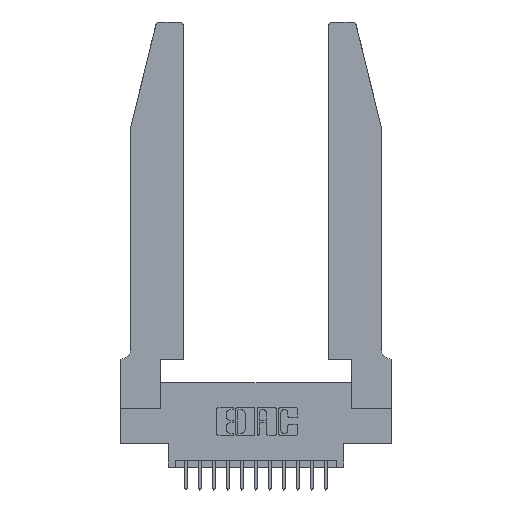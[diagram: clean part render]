
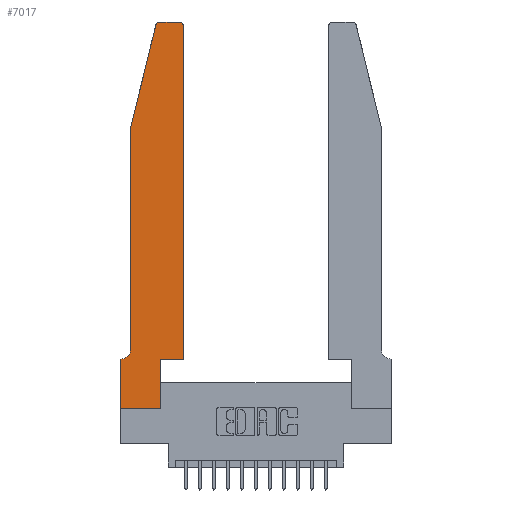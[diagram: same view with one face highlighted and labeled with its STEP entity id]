
A CAD part, top view. The second image highlights one B-rep face of the part: STEP entity #7017.
In plain terms, the highlighted planar face has unit normal (0, 0, 1).
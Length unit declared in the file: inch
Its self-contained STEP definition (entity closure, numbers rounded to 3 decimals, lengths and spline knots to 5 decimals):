
#17 = EDGE_CURVE ( 'NONE', #16693, #17585, #17739, .T. ) ;
#855 = CARTESIAN_POINT ( 'NONE',  ( 0.4505, 2.72, 0.37 ) ) ;
#924 = CARTESIAN_POINT ( 'NONE',  ( 0., 0., 0.37 ) ) ;
#1266 = CARTESIAN_POINT ( 'NONE',  ( 0.0755, 2., 0.37 ) ) ;
#1365 = CARTESIAN_POINT ( 'NONE',  ( 0.284, 2.75, 0.37 ) ) ;
#1381 = CARTESIAN_POINT ( 'NONE',  ( 0.4505, 0.35, 0.37 ) ) ;
#1466 = EDGE_CURVE ( 'NONE', #13858, #3915, #9994, .T. ) ;
#1896 = DIRECTION ( 'NONE',  ( 1., 0., 0. ) ) ;
#2001 = CARTESIAN_POINT ( 'NONE',  ( 0., 0., 0.37 ) ) ;
#2240 = DIRECTION ( 'NONE',  ( 0., 0., 1. ) ) ;
#2262 = DIRECTION ( 'NONE',  ( 0., 1., 0. ) ) ;
#3110 = CARTESIAN_POINT ( 'NONE',  ( 0.0755, 2., 0.37 ) ) ;
#3193 = ORIENTED_EDGE ( 'NONE', *, *, #17, .T. ) ;
#3297 = PLANE ( 'NONE',  #13897 ) ;
#3320 = DIRECTION ( 'NONE',  ( 1., 0., 0. ) ) ;
#3636 = ORIENTED_EDGE ( 'NONE', *, *, #8196, .T. ) ;
#3915 = VERTEX_POINT ( 'NONE', #15317 ) ;
#4298 = VERTEX_POINT ( 'NONE', #10493 ) ;
#4442 = CARTESIAN_POINT ( 'NONE',  ( 0.2865, 0., 0.37 ) ) ;
#4523 = CIRCLE ( 'NONE', #15562, 0.03 ) ;
#4702 = DIRECTION ( 'NONE',  ( 0., 0., 1. ) ) ;
#4775 = CARTESIAN_POINT ( 'NONE',  ( 0., 0.35, 0.37 ) ) ;
#5128 = LINE ( 'NONE', #2001, #5768 ) ;
#5158 = DIRECTION ( 'NONE',  ( -1., 0., 0. ) ) ;
#5293 = ORIENTED_EDGE ( 'NONE', *, *, #9450, .T. ) ;
#5401 = CARTESIAN_POINT ( 'NONE',  ( 0.2605, 2.75, 0.37 ) ) ;
#5768 = VECTOR ( 'NONE', #17195, 39.37008 ) ;
#6060 = LINE ( 'NONE', #14858, #16140 ) ;
#6226 = ORIENTED_EDGE ( 'NONE', *, *, #16073, .T. ) ;
#6567 = DIRECTION ( 'NONE',  ( 1., 0., 0. ) ) ;
#6626 = ORIENTED_EDGE ( 'NONE', *, *, #1466, .T. ) ;
#6933 = CARTESIAN_POINT ( 'NONE',  ( 0.4505, 0.35, 0.37 ) ) ;
#7017 = ADVANCED_FACE ( 'NONE', ( #11377 ), #3297, .T. ) ;
#7456 = DIRECTION ( 'NONE',  ( -1., 0., 0. ) ) ;
#7476 = EDGE_CURVE ( 'NONE', #12177, #15743, #13781, .T. ) ;
#7520 = DIRECTION ( 'NONE',  ( 1., 0., 0. ) ) ;
#7745 = VECTOR ( 'NONE', #3320, 39.37008 ) ;
#8021 = VECTOR ( 'NONE', #5158, 39.37008 ) ;
#8196 = EDGE_CURVE ( 'NONE', #17066, #16293, #16117, .T. ) ;
#8340 = ORIENTED_EDGE ( 'NONE', *, *, #13530, .T. ) ;
#8384 = LINE ( 'NONE', #16375, #7745 ) ;
#8445 = VERTEX_POINT ( 'NONE', #11913 ) ;
#8677 = DIRECTION ( 'NONE',  ( 0., 0., 1. ) ) ;
#8861 = EDGE_CURVE ( 'NONE', #15046, #17066, #13732, .T. ) ;
#8877 = DIRECTION ( 'NONE',  ( 0., 0., -1. ) ) ;
#8981 = ORIENTED_EDGE ( 'NONE', *, *, #7476, .T. ) ;
#9098 = CARTESIAN_POINT ( 'NONE',  ( 0.4205, 2.72, 0.37 ) ) ;
#9450 = EDGE_CURVE ( 'NONE', #15743, #16693, #5128, .T. ) ;
#9690 = CARTESIAN_POINT ( 'NONE',  ( 0., 0., 0.37 ) ) ;
#9819 = ORIENTED_EDGE ( 'NONE', *, *, #16255, .T. ) ;
#9908 = DIRECTION ( 'NONE',  ( 0., -1., 0. ) ) ;
#9994 = LINE ( 'NONE', #1266, #16200 ) ;
#10040 = CARTESIAN_POINT ( 'NONE',  ( 0.0055, 0.42, 0.37 ) ) ;
#10327 = DIRECTION ( 'NONE',  ( -1., 0., 0. ) ) ;
#10446 = AXIS2_PLACEMENT_3D ( 'NONE', #9098, #2240, #17386 ) ;
#10493 = CARTESIAN_POINT ( 'NONE',  ( 0.2865, 0.35, 0.37 ) ) ;
#10815 = DIRECTION ( 'NONE',  ( 0., 1., 0. ) ) ;
#11259 = AXIS2_PLACEMENT_3D ( 'NONE', #10040, #8877, #7456 ) ;
#11377 = FACE_OUTER_BOUND ( 'NONE', #15576, .T. ) ;
#11834 = VECTOR ( 'NONE', #10327, 39.37008 ) ;
#11913 = CARTESIAN_POINT ( 'NONE',  ( 0.25487, 2.72718, 0.37 ) ) ;
#11990 = ORIENTED_EDGE ( 'NONE', *, *, #8861, .T. ) ;
#12085 = ORIENTED_EDGE ( 'NONE', *, *, #14367, .T. ) ;
#12177 = VERTEX_POINT ( 'NONE', #16287 ) ;
#12669 = CARTESIAN_POINT ( 'NONE',  ( 0.0755, 0.35, 0.37 ) ) ;
#12782 = CARTESIAN_POINT ( 'NONE',  ( 0.284, 2.72, 0.37 ) ) ;
#12900 = CARTESIAN_POINT ( 'NONE',  ( 0.4205, 2.75, 0.37 ) ) ;
#13530 = EDGE_CURVE ( 'NONE', #3915, #12177, #17711, .T. ) ;
#13577 = EDGE_CURVE ( 'NONE', #17585, #4298, #13841, .T. ) ;
#13649 = ORIENTED_EDGE ( 'NONE', *, *, #14946, .T. ) ;
#13654 = DIRECTION ( 'NONE',  ( -0.239, -0.971, 0. ) ) ;
#13732 = LINE ( 'NONE', #1381, #16949 ) ;
#13781 = LINE ( 'NONE', #12669, #11834 ) ;
#13841 = LINE ( 'NONE', #14413, #15125 ) ;
#13858 = VERTEX_POINT ( 'NONE', #3110 ) ;
#13897 = AXIS2_PLACEMENT_3D ( 'NONE', #17058, #4702, #7520 ) ;
#14367 = EDGE_CURVE ( 'NONE', #16293, #15543, #17474, .T. ) ;
#14413 = CARTESIAN_POINT ( 'NONE',  ( 0.2865, 0.35, 0.37 ) ) ;
#14858 = CARTESIAN_POINT ( 'NONE',  ( 0.0755, 2., 0.37 ) ) ;
#14946 = EDGE_CURVE ( 'NONE', #8445, #13858, #6060, .T. ) ;
#15046 = VERTEX_POINT ( 'NONE', #6933 ) ;
#15125 = VECTOR ( 'NONE', #2262, 39.37008 ) ;
#15317 = CARTESIAN_POINT ( 'NONE',  ( 0.0755, 0.42, 0.37 ) ) ;
#15543 = VERTEX_POINT ( 'NONE', #1365 ) ;
#15562 = AXIS2_PLACEMENT_3D ( 'NONE', #12782, #8677, #1896 ) ;
#15576 = EDGE_LOOP ( 'NONE', ( #12085, #9819, #13649, #6626, #8340, #8981, #5293, #3193, #15713, #6226, #11990, #3636 ) ) ;
#15713 = ORIENTED_EDGE ( 'NONE', *, *, #13577, .T. ) ;
#15743 = VERTEX_POINT ( 'NONE', #4775 ) ;
#15781 = VECTOR ( 'NONE', #6567, 39.37008 ) ;
#16073 = EDGE_CURVE ( 'NONE', #4298, #15046, #8384, .T. ) ;
#16117 = CIRCLE ( 'NONE', #10446, 0.03 ) ;
#16140 = VECTOR ( 'NONE', #13654, 39.37008 ) ;
#16200 = VECTOR ( 'NONE', #9908, 39.37008 ) ;
#16255 = EDGE_CURVE ( 'NONE', #15543, #8445, #4523, .T. ) ;
#16287 = CARTESIAN_POINT ( 'NONE',  ( 0.0055, 0.35, 0.37 ) ) ;
#16293 = VERTEX_POINT ( 'NONE', #12900 ) ;
#16375 = CARTESIAN_POINT ( 'NONE',  ( 0.4505, 0.35, 0.37 ) ) ;
#16693 = VERTEX_POINT ( 'NONE', #9690 ) ;
#16949 = VECTOR ( 'NONE', #10815, 39.37008 ) ;
#17058 = CARTESIAN_POINT ( 'NONE',  ( 0., 0.35, 0.37 ) ) ;
#17066 = VERTEX_POINT ( 'NONE', #855 ) ;
#17195 = DIRECTION ( 'NONE',  ( 0., -1., 0. ) ) ;
#17386 = DIRECTION ( 'NONE',  ( 1., 0., 0. ) ) ;
#17474 = LINE ( 'NONE', #5401, #8021 ) ;
#17585 = VERTEX_POINT ( 'NONE', #4442 ) ;
#17711 = CIRCLE ( 'NONE', #11259, 0.07 ) ;
#17739 = LINE ( 'NONE', #924, #15781 ) ;
